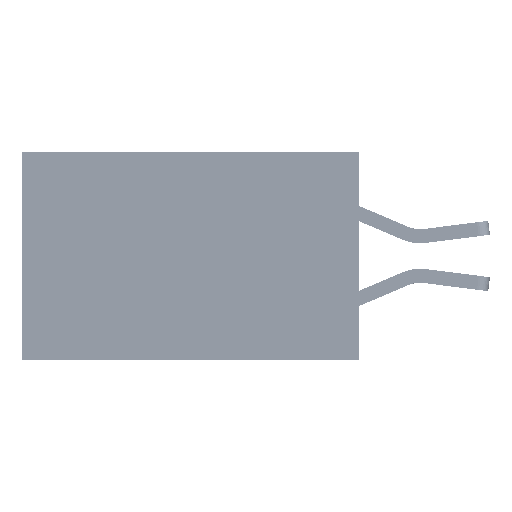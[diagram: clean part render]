
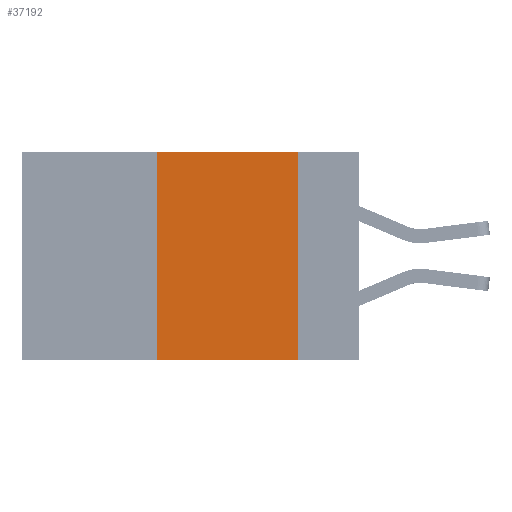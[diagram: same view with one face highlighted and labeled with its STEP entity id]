
A CAD part, left-side view. The second image highlights one B-rep face of the part: STEP entity #37192.
In plain terms, the highlighted planar face has unit normal (-1, 0, 0).
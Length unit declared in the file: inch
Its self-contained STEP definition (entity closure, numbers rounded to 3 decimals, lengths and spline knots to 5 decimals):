
#765 = CARTESIAN_POINT ( 'NONE',  ( 0., 0.11, 0. ) ) ;
#1190 = LINE ( 'NONE', #2810, #10486 ) ;
#2085 = ORIENTED_EDGE ( 'NONE', *, *, #29547, .F. ) ;
#2810 = CARTESIAN_POINT ( 'NONE',  ( 0., 0.6, 0. ) ) ;
#6113 = ORIENTED_EDGE ( 'NONE', *, *, #18282, .F. ) ;
#6844 = DIRECTION ( 'NONE',  ( 0., 0., -1. ) ) ;
#7809 = VERTEX_POINT ( 'NONE', #10659 ) ;
#10486 = VECTOR ( 'NONE', #29559, 39.37008 ) ;
#10659 = CARTESIAN_POINT ( 'NONE',  ( 0., 0.36, 0. ) ) ;
#11918 = FACE_OUTER_BOUND ( 'NONE', #25070, .T. ) ;
#12328 = DIRECTION ( 'NONE',  ( 0., -1., 0. ) ) ;
#16180 = ORIENTED_EDGE ( 'NONE', *, *, #22639, .T. ) ;
#16692 = AXIS2_PLACEMENT_3D ( 'NONE', #28005, #30851, #6844 ) ;
#16722 = VECTOR ( 'NONE', #18056, 39.37008 ) ;
#17224 = VERTEX_POINT ( 'NONE', #22265 ) ;
#17355 = LINE ( 'NONE', #17711, #23914 ) ;
#17711 = CARTESIAN_POINT ( 'NONE',  ( 0., 0.6, -0.37 ) ) ;
#18056 = DIRECTION ( 'NONE',  ( 0., 0., 1. ) ) ;
#18282 = EDGE_CURVE ( 'NONE', #34664, #7809, #29308, .T. ) ;
#18700 = LINE ( 'NONE', #765, #32237 ) ;
#22265 = CARTESIAN_POINT ( 'NONE',  ( 0., 0.11, 0. ) ) ;
#22639 = EDGE_CURVE ( 'NONE', #34664, #29115, #17355, .T. ) ;
#23431 = EDGE_CURVE ( 'NONE', #17224, #29115, #18700, .T. ) ;
#23914 = VECTOR ( 'NONE', #12328, 39.37008 ) ;
#24770 = CARTESIAN_POINT ( 'NONE',  ( 0., 0.11, -0.37 ) ) ;
#25070 = EDGE_LOOP ( 'NONE', ( #31608, #2085, #6113, #16180 ) ) ;
#27191 = CARTESIAN_POINT ( 'NONE',  ( 0., 0.36, 0. ) ) ;
#28005 = CARTESIAN_POINT ( 'NONE',  ( 0., 0.6, 0. ) ) ;
#29115 = VERTEX_POINT ( 'NONE', #24770 ) ;
#29308 = LINE ( 'NONE', #27191, #16722 ) ;
#29547 = EDGE_CURVE ( 'NONE', #7809, #17224, #1190, .T. ) ;
#29559 = DIRECTION ( 'NONE',  ( 0., -1., 0. ) ) ;
#30752 = DIRECTION ( 'NONE',  ( 0., 0., -1. ) ) ;
#30851 = DIRECTION ( 'NONE',  ( 1., 0., 0. ) ) ;
#31608 = ORIENTED_EDGE ( 'NONE', *, *, #23431, .F. ) ;
#32237 = VECTOR ( 'NONE', #30752, 39.37008 ) ;
#32903 = CARTESIAN_POINT ( 'NONE',  ( 0., 0.36, -0.37 ) ) ;
#34664 = VERTEX_POINT ( 'NONE', #32903 ) ;
#36728 = PLANE ( 'NONE',  #16692 ) ;
#37192 = ADVANCED_FACE ( 'NONE', ( #11918 ), #36728, .F. ) ;
